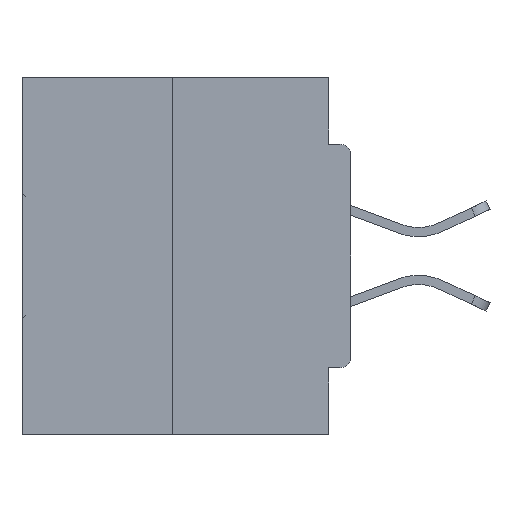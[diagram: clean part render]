
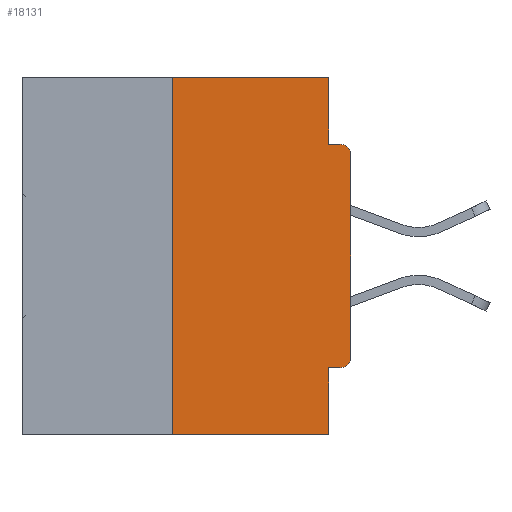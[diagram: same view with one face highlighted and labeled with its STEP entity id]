
A CAD part, left-side view. The second image highlights one B-rep face of the part: STEP entity #18131.
In plain terms, the highlighted planar face has unit normal (-1, 0, 0).
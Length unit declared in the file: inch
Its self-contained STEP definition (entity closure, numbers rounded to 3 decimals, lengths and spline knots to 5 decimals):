
#68 = CARTESIAN_POINT ( 'NONE',  ( 0., 0.46, 0. ) ) ;
#265 = AXIS2_PLACEMENT_3D ( 'NONE', #28277, #5163, #14813 ) ;
#358 = CARTESIAN_POINT ( 'NONE',  ( 0., 0., 0. ) ) ;
#607 = CARTESIAN_POINT ( 'NONE',  ( 0., 0., -0.0935 ) ) ;
#754 = FACE_OUTER_BOUND ( 'NONE', #15769, .T. ) ;
#1288 = LINE ( 'NONE', #14340, #21612 ) ;
#1692 = ORIENTED_EDGE ( 'NONE', *, *, #15813, .F. ) ;
#3569 = LINE ( 'NONE', #358, #15512 ) ;
#3830 = CARTESIAN_POINT ( 'NONE',  ( 0., 0.46, -0.5 ) ) ;
#4079 = CIRCLE ( 'NONE', #28025, 0.015 ) ;
#4171 = CARTESIAN_POINT ( 'NONE',  ( 0., 0.46, 0. ) ) ;
#4235 = DIRECTION ( 'NONE',  ( 0., -1., 0. ) ) ;
#5163 = DIRECTION ( 'NONE',  ( -1., 0., 0. ) ) ;
#5215 = AXIS2_PLACEMENT_3D ( 'NONE', #4171, #10593, #36906 ) ;
#5239 = ORIENTED_EDGE ( 'NONE', *, *, #14715, .T. ) ;
#6893 = VERTEX_POINT ( 'NONE', #18567 ) ;
#7963 = DIRECTION ( 'NONE',  ( 0., 1., 0. ) ) ;
#8441 = ORIENTED_EDGE ( 'NONE', *, *, #38897, .F. ) ;
#8782 = ORIENTED_EDGE ( 'NONE', *, *, #35312, .T. ) ;
#9318 = VERTEX_POINT ( 'NONE', #39482 ) ;
#9657 = LINE ( 'NONE', #19308, #19759 ) ;
#10218 = ORIENTED_EDGE ( 'NONE', *, *, #25634, .F. ) ;
#10593 = DIRECTION ( 'NONE',  ( 1., 0., 0. ) ) ;
#10851 = VECTOR ( 'NONE', #4235, 39.37008 ) ;
#12006 = EDGE_CURVE ( 'NONE', #6893, #13145, #26514, .T. ) ;
#12500 = DIRECTION ( 'NONE',  ( 0., -1., 0. ) ) ;
#13145 = VERTEX_POINT ( 'NONE', #19320 ) ;
#13417 = DIRECTION ( 'NONE',  ( 0., 0., 1. ) ) ;
#13441 = EDGE_CURVE ( 'NONE', #30368, #38359, #27863, .T. ) ;
#13579 = VECTOR ( 'NONE', #34471, 39.37008 ) ;
#13972 = CARTESIAN_POINT ( 'NONE',  ( 0., 0.25, -0.5 ) ) ;
#14340 = CARTESIAN_POINT ( 'NONE',  ( 0., 0.031, -0.5 ) ) ;
#14715 = EDGE_CURVE ( 'NONE', #34414, #13145, #4079, .T. ) ;
#14771 = CARTESIAN_POINT ( 'NONE',  ( 0., 0.015, -0.1085 ) ) ;
#14813 = DIRECTION ( 'NONE',  ( 0., 0., -1. ) ) ;
#15512 = VECTOR ( 'NONE', #13417, 39.37008 ) ;
#15564 = VERTEX_POINT ( 'NONE', #27325 ) ;
#15769 = EDGE_LOOP ( 'NONE', ( #1692, #40813, #18852, #10218, #29340, #41289, #8782, #5239, #23815, #8441 ) ) ;
#15813 = EDGE_CURVE ( 'NONE', #38359, #9318, #32161, .T. ) ;
#16092 = VECTOR ( 'NONE', #7963, 39.37008 ) ;
#16487 = LINE ( 'NONE', #3830, #33906 ) ;
#16909 = DIRECTION ( 'NONE',  ( 0., -1., 0. ) ) ;
#17274 = CARTESIAN_POINT ( 'NONE',  ( 0., 0.015, -0.4065 ) ) ;
#17356 = VECTOR ( 'NONE', #12500, 39.37008 ) ;
#17391 = EDGE_CURVE ( 'NONE', #31639, #24777, #26602, .T. ) ;
#18023 = CARTESIAN_POINT ( 'NONE',  ( 0., 0., -0.1085 ) ) ;
#18131 = ADVANCED_FACE ( 'NONE', ( #754 ), #40121, .F. ) ;
#18538 = CARTESIAN_POINT ( 'NONE',  ( 0., 0.25, 0. ) ) ;
#18557 = VERTEX_POINT ( 'NONE', #38036 ) ;
#18567 = CARTESIAN_POINT ( 'NONE',  ( 0., 0.031, -0.0935 ) ) ;
#18852 = ORIENTED_EDGE ( 'NONE', *, *, #34828, .T. ) ;
#19308 = CARTESIAN_POINT ( 'NONE',  ( 0., 0.031, 0. ) ) ;
#19320 = CARTESIAN_POINT ( 'NONE',  ( 0., 0.015, -0.0935 ) ) ;
#19759 = VECTOR ( 'NONE', #25961, 39.37008 ) ;
#21612 = VECTOR ( 'NONE', #40632, 39.37008 ) ;
#23703 = EDGE_CURVE ( 'NONE', #31639, #18557, #41971, .T. ) ;
#23815 = ORIENTED_EDGE ( 'NONE', *, *, #12006, .F. ) ;
#24777 = VERTEX_POINT ( 'NONE', #40371 ) ;
#25634 = EDGE_CURVE ( 'NONE', #24777, #15564, #1288, .T. ) ;
#25961 = DIRECTION ( 'NONE',  ( 0., 0., -1. ) ) ;
#26514 = LINE ( 'NONE', #607, #10851 ) ;
#26602 = LINE ( 'NONE', #33850, #16092 ) ;
#27325 = CARTESIAN_POINT ( 'NONE',  ( 0., 0.031, -0.5 ) ) ;
#27830 = DIRECTION ( 'NONE',  ( 0., 0., -1. ) ) ;
#27863 = LINE ( 'NONE', #40902, #13579 ) ;
#28025 = AXIS2_PLACEMENT_3D ( 'NONE', #14771, #36205, #27830 ) ;
#28277 = CARTESIAN_POINT ( 'NONE',  ( 0., 0.015, -0.3915 ) ) ;
#29340 = ORIENTED_EDGE ( 'NONE', *, *, #17391, .F. ) ;
#30368 = VERTEX_POINT ( 'NONE', #13972 ) ;
#31639 = VERTEX_POINT ( 'NONE', #17274 ) ;
#32161 = LINE ( 'NONE', #68, #17356 ) ;
#33850 = CARTESIAN_POINT ( 'NONE',  ( 0., 0., -0.4065 ) ) ;
#33906 = VECTOR ( 'NONE', #16909, 39.37008 ) ;
#34414 = VERTEX_POINT ( 'NONE', #18023 ) ;
#34471 = DIRECTION ( 'NONE',  ( 0., 0., 1. ) ) ;
#34828 = EDGE_CURVE ( 'NONE', #30368, #15564, #16487, .T. ) ;
#35312 = EDGE_CURVE ( 'NONE', #18557, #34414, #3569, .T. ) ;
#36205 = DIRECTION ( 'NONE',  ( -1., 0., 0. ) ) ;
#36906 = DIRECTION ( 'NONE',  ( 0., 0., -1. ) ) ;
#38036 = CARTESIAN_POINT ( 'NONE',  ( 0., 0., -0.3915 ) ) ;
#38359 = VERTEX_POINT ( 'NONE', #18538 ) ;
#38897 = EDGE_CURVE ( 'NONE', #9318, #6893, #9657, .T. ) ;
#39482 = CARTESIAN_POINT ( 'NONE',  ( 0., 0.031, 0. ) ) ;
#40121 = PLANE ( 'NONE',  #5215 ) ;
#40371 = CARTESIAN_POINT ( 'NONE',  ( 0., 0.031, -0.4065 ) ) ;
#40632 = DIRECTION ( 'NONE',  ( 0., 0., -1. ) ) ;
#40813 = ORIENTED_EDGE ( 'NONE', *, *, #13441, .F. ) ;
#40902 = CARTESIAN_POINT ( 'NONE',  ( 0., 0.25, 0. ) ) ;
#41289 = ORIENTED_EDGE ( 'NONE', *, *, #23703, .T. ) ;
#41971 = CIRCLE ( 'NONE', #265, 0.015 ) ;
